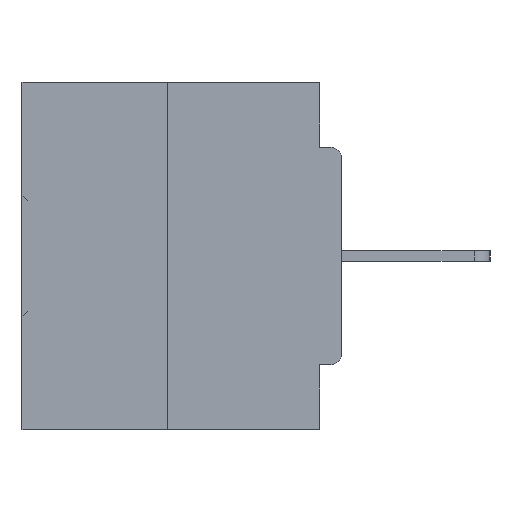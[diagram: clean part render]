
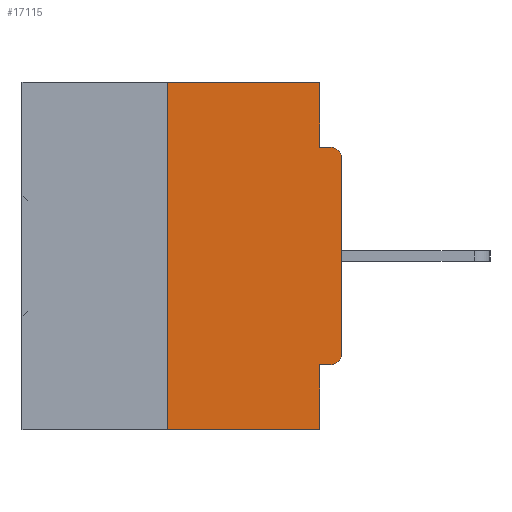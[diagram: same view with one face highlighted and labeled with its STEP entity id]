
A CAD part, left-side view. The second image highlights one B-rep face of the part: STEP entity #17115.
In plain terms, the highlighted planar face has unit normal (-1, 0, 0).
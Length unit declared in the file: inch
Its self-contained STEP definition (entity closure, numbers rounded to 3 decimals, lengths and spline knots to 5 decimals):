
#1309 = VECTOR ( 'NONE', #10370, 39.37008 ) ;
#1349 = DIRECTION ( 'NONE',  ( 0., 0., 1. ) ) ;
#1747 = LINE ( 'NONE', #23382, #24096 ) ;
#2019 = ORIENTED_EDGE ( 'NONE', *, *, #14084, .F. ) ;
#2229 = CARTESIAN_POINT ( 'NONE',  ( 0., 0.25, -0.5 ) ) ;
#2608 = LINE ( 'NONE', #17903, #37349 ) ;
#2946 = VECTOR ( 'NONE', #1349, 39.37008 ) ;
#3738 = VERTEX_POINT ( 'NONE', #12158 ) ;
#5670 = DIRECTION ( 'NONE',  ( -1., 0., 0. ) ) ;
#6062 = EDGE_CURVE ( 'NONE', #6129, #18929, #32430, .T. ) ;
#6129 = VERTEX_POINT ( 'NONE', #2229 ) ;
#6564 = AXIS2_PLACEMENT_3D ( 'NONE', #36124, #23470, #8568 ) ;
#6944 = ORIENTED_EDGE ( 'NONE', *, *, #28590, .T. ) ;
#6964 = LINE ( 'NONE', #25314, #35379 ) ;
#7177 = VECTOR ( 'NONE', #27028, 39.37008 ) ;
#8512 = EDGE_CURVE ( 'NONE', #3738, #17508, #19104, .T. ) ;
#8568 = DIRECTION ( 'NONE',  ( 0., 0., -1. ) ) ;
#9930 = EDGE_CURVE ( 'NONE', #15602, #31958, #35632, .T. ) ;
#10067 = EDGE_LOOP ( 'NONE', ( #2019, #11580, #24301, #34676, #11067, #6944, #28804, #22000, #21739, #19580 ) ) ;
#10370 = DIRECTION ( 'NONE',  ( 0., 1., 0. ) ) ;
#11067 = ORIENTED_EDGE ( 'NONE', *, *, #40314, .F. ) ;
#11114 = DIRECTION ( 'NONE',  ( -1., 0., 0. ) ) ;
#11399 = CARTESIAN_POINT ( 'NONE',  ( 0., 0.25, 0. ) ) ;
#11580 = ORIENTED_EDGE ( 'NONE', *, *, #29756, .F. ) ;
#11623 = EDGE_CURVE ( 'NONE', #31958, #18969, #33698, .T. ) ;
#12158 = CARTESIAN_POINT ( 'NONE',  ( 0., 0.031, 0. ) ) ;
#13014 = CARTESIAN_POINT ( 'NONE',  ( 0., 0., -0.3915 ) ) ;
#13142 = CARTESIAN_POINT ( 'NONE',  ( 0., 0., -0.1085 ) ) ;
#13689 = DIRECTION ( 'NONE',  ( 0., -1., 0. ) ) ;
#14084 = EDGE_CURVE ( 'NONE', #35463, #3738, #1747, .T. ) ;
#14203 = DIRECTION ( 'NONE',  ( 0., -1., 0. ) ) ;
#14262 = DIRECTION ( 'NONE',  ( 0., 0., 1. ) ) ;
#14584 = CARTESIAN_POINT ( 'NONE',  ( 0., 0., -0.0935 ) ) ;
#15056 = CARTESIAN_POINT ( 'NONE',  ( 0., 0.031, -0.5 ) ) ;
#15602 = VERTEX_POINT ( 'NONE', #13014 ) ;
#15661 = CARTESIAN_POINT ( 'NONE',  ( 0., 0.015, -0.0935 ) ) ;
#16302 = EDGE_CURVE ( 'NONE', #17508, #18969, #26628, .T. ) ;
#17115 = ADVANCED_FACE ( 'NONE', ( #23669 ), #39181, .F. ) ;
#17508 = VERTEX_POINT ( 'NONE', #33181 ) ;
#17903 = CARTESIAN_POINT ( 'NONE',  ( 0., 0.25, 0. ) ) ;
#18929 = VERTEX_POINT ( 'NONE', #15056 ) ;
#18969 = VERTEX_POINT ( 'NONE', #15661 ) ;
#19104 = LINE ( 'NONE', #25228, #30957 ) ;
#19580 = ORIENTED_EDGE ( 'NONE', *, *, #8512, .F. ) ;
#20575 = DIRECTION ( 'NONE',  ( 0., 0., -1. ) ) ;
#21739 = ORIENTED_EDGE ( 'NONE', *, *, #16302, .F. ) ;
#22000 = ORIENTED_EDGE ( 'NONE', *, *, #11623, .T. ) ;
#22165 = DIRECTION ( 'NONE',  ( 0., 0., -1. ) ) ;
#23198 = CARTESIAN_POINT ( 'NONE',  ( 0., 0., -0.4065 ) ) ;
#23382 = CARTESIAN_POINT ( 'NONE',  ( 0., 0.46, 0. ) ) ;
#23470 = DIRECTION ( 'NONE',  ( 1., 0., 0. ) ) ;
#23548 = DIRECTION ( 'NONE',  ( 0., 0., -1. ) ) ;
#23669 = FACE_OUTER_BOUND ( 'NONE', #10067, .T. ) ;
#24096 = VECTOR ( 'NONE', #14203, 39.37008 ) ;
#24301 = ORIENTED_EDGE ( 'NONE', *, *, #6062, .T. ) ;
#25099 = CARTESIAN_POINT ( 'NONE',  ( 0., 0.031, -0.4065 ) ) ;
#25228 = CARTESIAN_POINT ( 'NONE',  ( 0., 0.031, 0. ) ) ;
#25314 = CARTESIAN_POINT ( 'NONE',  ( 0., 0.031, -0.5 ) ) ;
#25593 = VECTOR ( 'NONE', #13689, 39.37008 ) ;
#26119 = DIRECTION ( 'NONE',  ( 0., 0., -1. ) ) ;
#26448 = CARTESIAN_POINT ( 'NONE',  ( 0., 0., 0. ) ) ;
#26609 = CARTESIAN_POINT ( 'NONE',  ( 0., 0.015, -0.1085 ) ) ;
#26628 = LINE ( 'NONE', #14584, #7177 ) ;
#26811 = EDGE_CURVE ( 'NONE', #29568, #18929, #6964, .T. ) ;
#27028 = DIRECTION ( 'NONE',  ( 0., -1., 0. ) ) ;
#27555 = VERTEX_POINT ( 'NONE', #27870 ) ;
#27870 = CARTESIAN_POINT ( 'NONE',  ( 0., 0.015, -0.4065 ) ) ;
#28590 = EDGE_CURVE ( 'NONE', #27555, #15602, #34185, .T. ) ;
#28804 = ORIENTED_EDGE ( 'NONE', *, *, #9930, .T. ) ;
#29385 = CARTESIAN_POINT ( 'NONE',  ( 0., 0.46, -0.5 ) ) ;
#29568 = VERTEX_POINT ( 'NONE', #25099 ) ;
#29756 = EDGE_CURVE ( 'NONE', #6129, #35463, #2608, .T. ) ;
#30957 = VECTOR ( 'NONE', #22165, 39.37008 ) ;
#31958 = VERTEX_POINT ( 'NONE', #13142 ) ;
#32368 = LINE ( 'NONE', #23198, #1309 ) ;
#32430 = LINE ( 'NONE', #29385, #25593 ) ;
#33181 = CARTESIAN_POINT ( 'NONE',  ( 0., 0.031, -0.0935 ) ) ;
#33608 = CARTESIAN_POINT ( 'NONE',  ( 0., 0.015, -0.3915 ) ) ;
#33698 = CIRCLE ( 'NONE', #40213, 0.015 ) ;
#34185 = CIRCLE ( 'NONE', #39400, 0.015 ) ;
#34676 = ORIENTED_EDGE ( 'NONE', *, *, #26811, .F. ) ;
#35379 = VECTOR ( 'NONE', #26119, 39.37008 ) ;
#35463 = VERTEX_POINT ( 'NONE', #11399 ) ;
#35632 = LINE ( 'NONE', #26448, #2946 ) ;
#36124 = CARTESIAN_POINT ( 'NONE',  ( 0., 0.46, 0. ) ) ;
#37349 = VECTOR ( 'NONE', #14262, 39.37008 ) ;
#39181 = PLANE ( 'NONE',  #6564 ) ;
#39400 = AXIS2_PLACEMENT_3D ( 'NONE', #33608, #5670, #20575 ) ;
#40213 = AXIS2_PLACEMENT_3D ( 'NONE', #26609, #11114, #23548 ) ;
#40314 = EDGE_CURVE ( 'NONE', #27555, #29568, #32368, .T. ) ;
